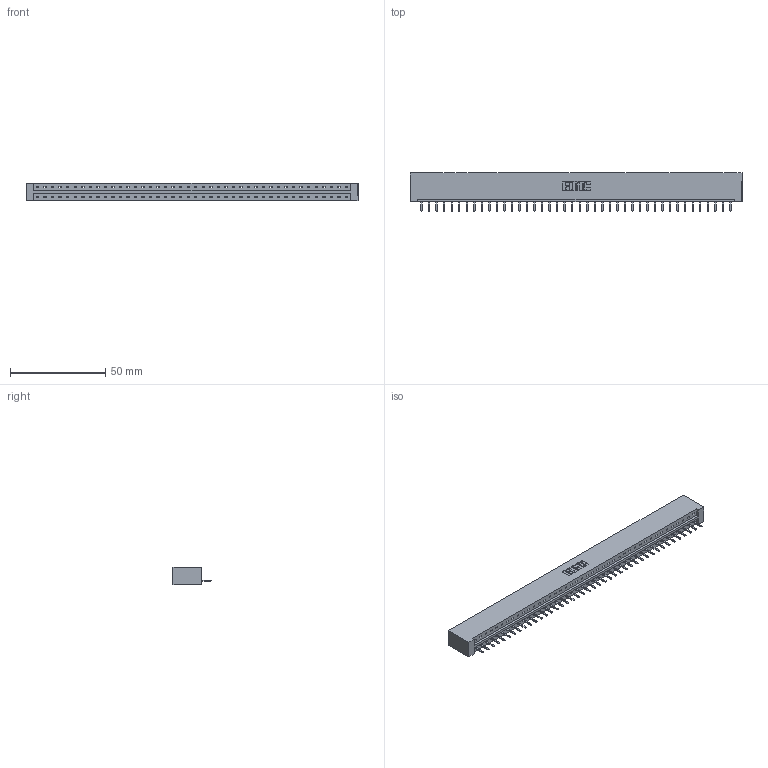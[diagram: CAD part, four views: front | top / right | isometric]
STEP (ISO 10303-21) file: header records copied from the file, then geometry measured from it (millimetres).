
FILE_DESCRIPTION (( 'STEP AP203' ), '1' );
FILE_NAME ('833-042-520-101.STEP', '2020-06-03T20:07:07', ( '' ), ( '' ), 'SwSTEP 2.0', 'SolidWorks 2020', '' );
FILE_SCHEMA (( 'CONFIG_CONTROL_DESIGN' ));
Length unit declared in the file: inch
Products named in the file (3): 833 Part_Lugless; 345-292-001_345-293-120; 833-042-520-101
Assembly tree (43 placements, depth 2):
  833-042-520-101
    833 Part_Lugless
    345-292-001_345-293-120  x42
Bounding box: 174.68 x 20.02 x 9.4 mm (x, y, z)
Volume: 18069.2 mm3; surface area: 19083.4 mm2
Topology: 43 solids, 43 shells, 2710 faces, 8015 edges, 5230 vertices
Faces by surface type: plane 1914, cylinder 796
Entity records: 25513 total; most frequent: CARTESIAN_POINT 4420, ORIENTED_EDGE 4386, DIRECTION 3709, EDGE_CURVE 2193, LINE 2069, VECTOR 2069, VERTEX_POINT 1458, AXIS2_PLACEMENT_3D 820
